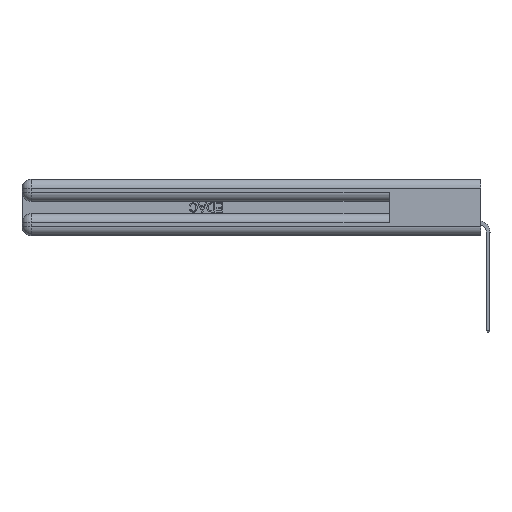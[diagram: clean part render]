
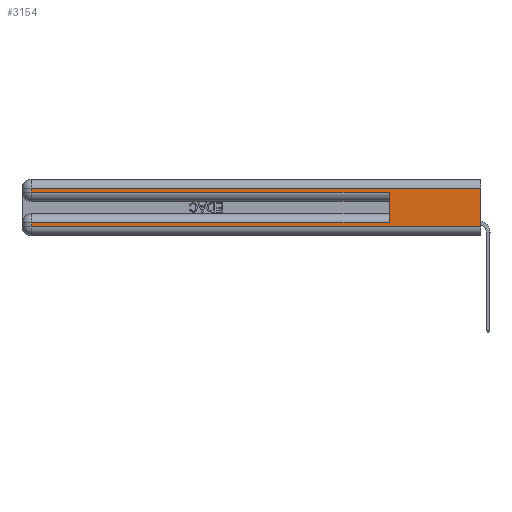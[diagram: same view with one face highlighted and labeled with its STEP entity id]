
A CAD part, left-side view. The second image highlights one B-rep face of the part: STEP entity #3154.
In plain terms, the highlighted planar face has unit normal (-1, 0, 0).
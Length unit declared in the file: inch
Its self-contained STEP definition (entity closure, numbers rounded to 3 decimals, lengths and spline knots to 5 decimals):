
#284 = VERTEX_POINT ( 'NONE', #34078 ) ;
#1057 = DIRECTION ( 'NONE',  ( 0., 0., 1. ) ) ;
#1432 = EDGE_CURVE ( 'NONE', #4636, #25449, #30605, .T. ) ;
#1744 = VERTEX_POINT ( 'NONE', #24814 ) ;
#1783 = PLANE ( 'NONE',  #22590 ) ;
#1938 = DIRECTION ( 'NONE',  ( 0., 0., -1. ) ) ;
#3154 = ADVANCED_FACE ( 'NONE', ( #41447 ), #1783, .F. ) ;
#3183 = VECTOR ( 'NONE', #14629, 39.37008 ) ;
#3617 = DIRECTION ( 'NONE',  ( 0., 1., 0. ) ) ;
#3621 = EDGE_CURVE ( 'NONE', #10287, #37506, #31890, .T. ) ;
#4435 = CARTESIAN_POINT ( 'NONE',  ( 0., 0., 0.06 ) ) ;
#4636 = VERTEX_POINT ( 'NONE', #16519 ) ;
#4811 = DIRECTION ( 'NONE',  ( 0., -1., 0. ) ) ;
#5416 = VECTOR ( 'NONE', #3617, 39.37008 ) ;
#6439 = CARTESIAN_POINT ( 'NONE',  ( 0., 2.94, 0.06 ) ) ;
#7608 = ORIENTED_EDGE ( 'NONE', *, *, #31054, .F. ) ;
#8535 = CARTESIAN_POINT ( 'NONE',  ( 0., 0., 0.37 ) ) ;
#9194 = CARTESIAN_POINT ( 'NONE',  ( 0., 0., 0.31 ) ) ;
#10287 = VERTEX_POINT ( 'NONE', #17179 ) ;
#10536 = CARTESIAN_POINT ( 'NONE',  ( 0., 0., 0.085 ) ) ;
#10842 = EDGE_CURVE ( 'NONE', #37506, #1744, #24223, .T. ) ;
#11473 = ORIENTED_EDGE ( 'NONE', *, *, #29784, .T. ) ;
#12846 = DIRECTION ( 'NONE',  ( 0., 1., 0. ) ) ;
#13218 = CARTESIAN_POINT ( 'NONE',  ( 0., 2.94, 0.37 ) ) ;
#13820 = VECTOR ( 'NONE', #42687, 39.37008 ) ;
#14629 = DIRECTION ( 'NONE',  ( 0., -1., 0. ) ) ;
#14681 = CARTESIAN_POINT ( 'NONE',  ( 0., 0.6, 0.145 ) ) ;
#15207 = VERTEX_POINT ( 'NONE', #17742 ) ;
#16519 = CARTESIAN_POINT ( 'NONE',  ( 0., 2.94, 0.285 ) ) ;
#16569 = CARTESIAN_POINT ( 'NONE',  ( 0., 2.94, 0.37 ) ) ;
#17179 = CARTESIAN_POINT ( 'NONE',  ( 0., 2.94, 0.085 ) ) ;
#17742 = CARTESIAN_POINT ( 'NONE',  ( 0., 2.94, 0.31 ) ) ;
#17920 = EDGE_CURVE ( 'NONE', #26888, #1744, #34819, .T. ) ;
#19542 = VECTOR ( 'NONE', #4811, 39.37008 ) ;
#20345 = ORIENTED_EDGE ( 'NONE', *, *, #1432, .T. ) ;
#21701 = CARTESIAN_POINT ( 'NONE',  ( 0., 0., 0.37 ) ) ;
#22590 = AXIS2_PLACEMENT_3D ( 'NONE', #21701, #31701, #1938 ) ;
#24223 = LINE ( 'NONE', #4435, #3183 ) ;
#24559 = VECTOR ( 'NONE', #31473, 39.37008 ) ;
#24814 = CARTESIAN_POINT ( 'NONE',  ( 0., 0., 0.06 ) ) ;
#24999 = CARTESIAN_POINT ( 'NONE',  ( 0., 0., 0.285 ) ) ;
#25449 = VERTEX_POINT ( 'NONE', #38483 ) ;
#26888 = VERTEX_POINT ( 'NONE', #9194 ) ;
#26980 = VECTOR ( 'NONE', #33322, 39.37008 ) ;
#27701 = ORIENTED_EDGE ( 'NONE', *, *, #39328, .T. ) ;
#27988 = LINE ( 'NONE', #13218, #26980 ) ;
#29657 = VECTOR ( 'NONE', #12846, 39.37008 ) ;
#29784 = EDGE_CURVE ( 'NONE', #284, #10287, #35451, .T. ) ;
#30605 = LINE ( 'NONE', #24999, #19542 ) ;
#31054 = EDGE_CURVE ( 'NONE', #284, #25449, #39581, .T. ) ;
#31473 = DIRECTION ( 'NONE',  ( 0., 0., -1. ) ) ;
#31701 = DIRECTION ( 'NONE',  ( 1., 0., 0. ) ) ;
#31890 = LINE ( 'NONE', #16569, #24559 ) ;
#33322 = DIRECTION ( 'NONE',  ( 0., 0., -1. ) ) ;
#34078 = CARTESIAN_POINT ( 'NONE',  ( 0., 0.6, 0.085 ) ) ;
#34252 = VECTOR ( 'NONE', #1057, 39.37008 ) ;
#34819 = LINE ( 'NONE', #8535, #13820 ) ;
#35425 = LINE ( 'NONE', #43595, #29657 ) ;
#35451 = LINE ( 'NONE', #10536, #5416 ) ;
#35787 = ORIENTED_EDGE ( 'NONE', *, *, #38676, .T. ) ;
#36754 = ORIENTED_EDGE ( 'NONE', *, *, #3621, .T. ) ;
#37030 = ORIENTED_EDGE ( 'NONE', *, *, #10842, .T. ) ;
#37506 = VERTEX_POINT ( 'NONE', #6439 ) ;
#38483 = CARTESIAN_POINT ( 'NONE',  ( 0., 0.6, 0.285 ) ) ;
#38676 = EDGE_CURVE ( 'NONE', #26888, #15207, #35425, .T. ) ;
#39328 = EDGE_CURVE ( 'NONE', #15207, #4636, #27988, .T. ) ;
#39581 = LINE ( 'NONE', #14681, #34252 ) ;
#40337 = EDGE_LOOP ( 'NONE', ( #42190, #35787, #27701, #20345, #7608, #11473, #36754, #37030 ) ) ;
#41447 = FACE_OUTER_BOUND ( 'NONE', #40337, .T. ) ;
#42190 = ORIENTED_EDGE ( 'NONE', *, *, #17920, .F. ) ;
#42687 = DIRECTION ( 'NONE',  ( 0., 0., -1. ) ) ;
#43595 = CARTESIAN_POINT ( 'NONE',  ( 0., 0., 0.31 ) ) ;
